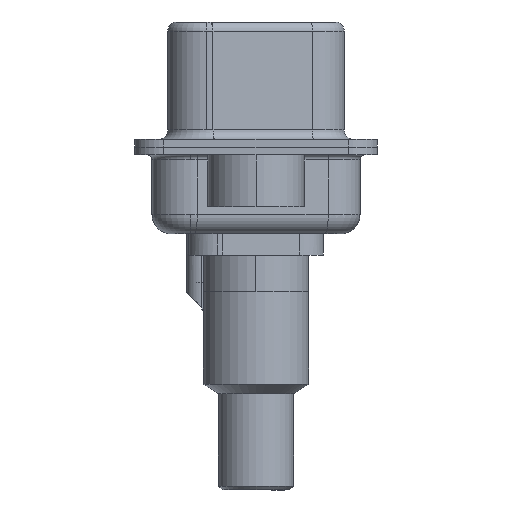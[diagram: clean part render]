
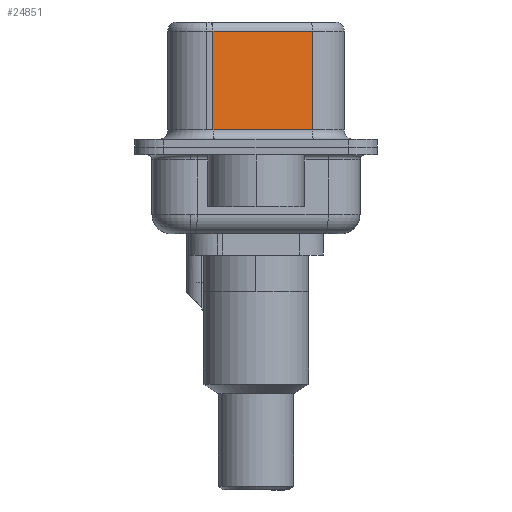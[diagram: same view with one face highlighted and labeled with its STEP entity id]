
A CAD part, left-side view. The second image highlights one B-rep face of the part: STEP entity #24851.
In plain terms, the highlighted planar face has unit normal (-0.985, -0.174, 0).
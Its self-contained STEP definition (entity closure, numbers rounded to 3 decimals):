
#713 = DIRECTION ( 'NONE',  ( 0., 0., -1. ) ) ;
#758 = DIRECTION ( 'NONE',  ( 0., 0., -1. ) ) ;
#1210 = DIRECTION ( 'NONE',  ( 0.985, 0.174, 0. ) ) ;
#1912 = ORIENTED_EDGE ( 'NONE', *, *, #3067, .T. ) ;
#3067 = EDGE_CURVE ( 'NONE', #6235, #6553, #9860, .T. ) ;
#3594 = CARTESIAN_POINT ( 'NONE',  ( 4.58, -2.927, 0.9 ) ) ;
#3710 = LINE ( 'NONE', #14932, #24804 ) ;
#4487 = VECTOR ( 'NONE', #16486, 1000. ) ;
#5203 = ORIENTED_EDGE ( 'NONE', *, *, #23971, .T. ) ;
#5811 = EDGE_CURVE ( 'NONE', #22421, #18651, #12637, .T. ) ;
#6235 = VERTEX_POINT ( 'NONE', #11887 ) ;
#6553 = VERTEX_POINT ( 'NONE', #9046 ) ;
#7833 = ORIENTED_EDGE ( 'NONE', *, *, #9861, .F. ) ;
#9046 = CARTESIAN_POINT ( 'NONE',  ( 3.67, 2.233, 6.02 ) ) ;
#9860 = LINE ( 'NONE', #26379, #4487 ) ;
#9861 = EDGE_CURVE ( 'NONE', #6235, #18651, #23758, .T. ) ;
#11327 = PLANE ( 'NONE',  #12239 ) ;
#11887 = CARTESIAN_POINT ( 'NONE',  ( 4.58, -2.927, 6.02 ) ) ;
#12239 = AXIS2_PLACEMENT_3D ( 'NONE', #25667, #1210, #15427 ) ;
#12614 = DIRECTION ( 'NONE',  ( 0.174, -0.985, 0. ) ) ;
#12637 = LINE ( 'NONE', #20808, #22973 ) ;
#12667 = CARTESIAN_POINT ( 'NONE',  ( 3.67, 2.233, 0.9 ) ) ;
#12709 = ORIENTED_EDGE ( 'NONE', *, *, #5811, .T. ) ;
#12775 = VECTOR ( 'NONE', #758, 1000. ) ;
#14932 = CARTESIAN_POINT ( 'NONE',  ( 3.67, 2.233, 6.52 ) ) ;
#14975 = CARTESIAN_POINT ( 'NONE',  ( 4.58, -2.927, 6.52 ) ) ;
#15427 = DIRECTION ( 'NONE',  ( -0.174, 0.985, 0. ) ) ;
#16486 = DIRECTION ( 'NONE',  ( -0.174, 0.985, 0. ) ) ;
#18651 = VERTEX_POINT ( 'NONE', #3594 ) ;
#20808 = CARTESIAN_POINT ( 'NONE',  ( 4.58, -2.927, 0.9 ) ) ;
#22421 = VERTEX_POINT ( 'NONE', #12667 ) ;
#22973 = VECTOR ( 'NONE', #12614, 1000. ) ;
#23758 = LINE ( 'NONE', #14975, #12775 ) ;
#23971 = EDGE_CURVE ( 'NONE', #6553, #22421, #3710, .T. ) ;
#24804 = VECTOR ( 'NONE', #713, 1000. ) ;
#24851 = ADVANCED_FACE ( 'NONE', ( #25717 ), #11327, .F. ) ;
#25336 = EDGE_LOOP ( 'NONE', ( #7833, #1912, #5203, #12709 ) ) ;
#25667 = CARTESIAN_POINT ( 'NONE',  ( 4.58, -2.927, 6.52 ) ) ;
#25717 = FACE_OUTER_BOUND ( 'NONE', #25336, .T. ) ;
#26379 = CARTESIAN_POINT ( 'NONE',  ( 4.58, -2.927, 6.02 ) ) ;
